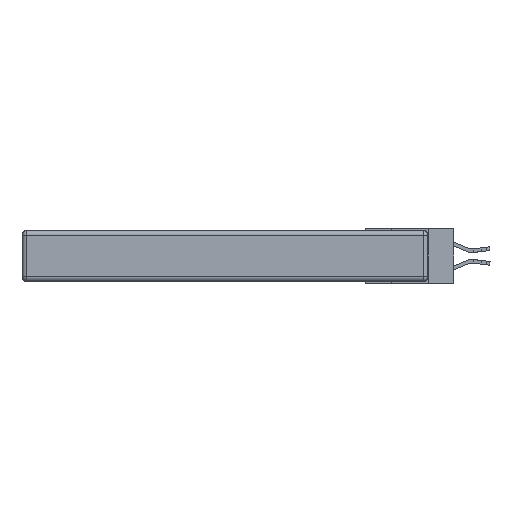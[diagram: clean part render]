
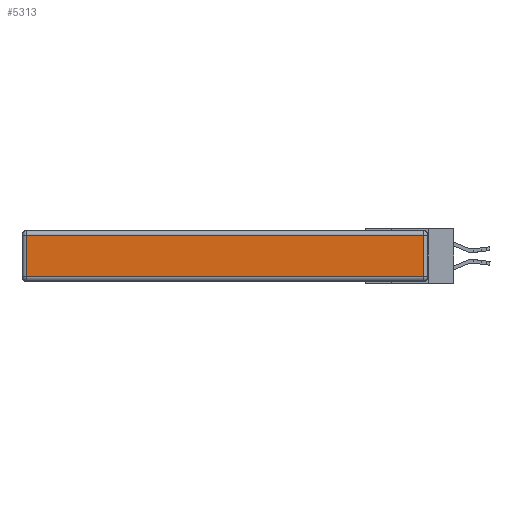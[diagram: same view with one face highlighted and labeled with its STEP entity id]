
A CAD part, left-side view. The second image highlights one B-rep face of the part: STEP entity #5313.
In plain terms, the highlighted planar face has unit normal (-1, 0, 0).
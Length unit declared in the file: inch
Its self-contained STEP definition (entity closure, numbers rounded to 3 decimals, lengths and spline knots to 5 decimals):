
#653 = DIRECTION ( 'NONE',  ( -1., 0., 0. ) ) ;
#742 = DIRECTION ( 'NONE',  ( 0., 0., 1. ) ) ;
#888 = VERTEX_POINT ( 'NONE', #20255 ) ;
#2457 = VECTOR ( 'NONE', #16165, 39.37008 ) ;
#2931 = DIRECTION ( 'NONE',  ( 0., 0., 1. ) ) ;
#4644 = FACE_OUTER_BOUND ( 'NONE', #11390, .T. ) ;
#4971 = EDGE_CURVE ( 'NONE', #22557, #888, #23748, .T. ) ;
#5313 = ADVANCED_FACE ( 'NONE', ( #4644 ), #21320, .T. ) ;
#5379 = DIRECTION ( 'NONE',  ( 0., 0., -1. ) ) ;
#7000 = VECTOR ( 'NONE', #7064, 39.37008 ) ;
#7064 = DIRECTION ( 'NONE',  ( 0., 1., 0. ) ) ;
#8164 = ORIENTED_EDGE ( 'NONE', *, *, #4971, .T. ) ;
#8766 = LINE ( 'NONE', #11848, #7000 ) ;
#9477 = AXIS2_PLACEMENT_3D ( 'NONE', #27874, #653, #2931 ) ;
#10274 = LINE ( 'NONE', #20678, #2457 ) ;
#11390 = EDGE_LOOP ( 'NONE', ( #26739, #12968, #15652, #8164 ) ) ;
#11848 = CARTESIAN_POINT ( 'NONE',  ( 0., 2.75, -0.03 ) ) ;
#12141 = CARTESIAN_POINT ( 'NONE',  ( 0., 2.72, -0.343 ) ) ;
#12241 = CARTESIAN_POINT ( 'NONE',  ( 0., 2.72, -0.03 ) ) ;
#12458 = VECTOR ( 'NONE', #742, 39.37008 ) ;
#12968 = ORIENTED_EDGE ( 'NONE', *, *, #26177, .T. ) ;
#13721 = CARTESIAN_POINT ( 'NONE',  ( 0., 0.03, -0.313 ) ) ;
#15652 = ORIENTED_EDGE ( 'NONE', *, *, #28094, .T. ) ;
#16165 = DIRECTION ( 'NONE',  ( 0., -1., 0. ) ) ;
#17033 = VECTOR ( 'NONE', #5379, 39.37008 ) ;
#18135 = VERTEX_POINT ( 'NONE', #23098 ) ;
#20255 = CARTESIAN_POINT ( 'NONE',  ( 0., 2.72, -0.313 ) ) ;
#20678 = CARTESIAN_POINT ( 'NONE',  ( 0., 0., -0.313 ) ) ;
#21004 = CARTESIAN_POINT ( 'NONE',  ( 0., 0.03, -0.343 ) ) ;
#21320 = PLANE ( 'NONE',  #9477 ) ;
#22557 = VERTEX_POINT ( 'NONE', #12241 ) ;
#23019 = LINE ( 'NONE', #21004, #12458 ) ;
#23098 = CARTESIAN_POINT ( 'NONE',  ( 0., 0.03, -0.03 ) ) ;
#23748 = LINE ( 'NONE', #12141, #17033 ) ;
#26177 = EDGE_CURVE ( 'NONE', #26326, #18135, #23019, .T. ) ;
#26326 = VERTEX_POINT ( 'NONE', #13721 ) ;
#26477 = EDGE_CURVE ( 'NONE', #888, #26326, #10274, .T. ) ;
#26739 = ORIENTED_EDGE ( 'NONE', *, *, #26477, .T. ) ;
#27874 = CARTESIAN_POINT ( 'NONE',  ( 0., 0., -0.343 ) ) ;
#28094 = EDGE_CURVE ( 'NONE', #18135, #22557, #8766, .T. ) ;
